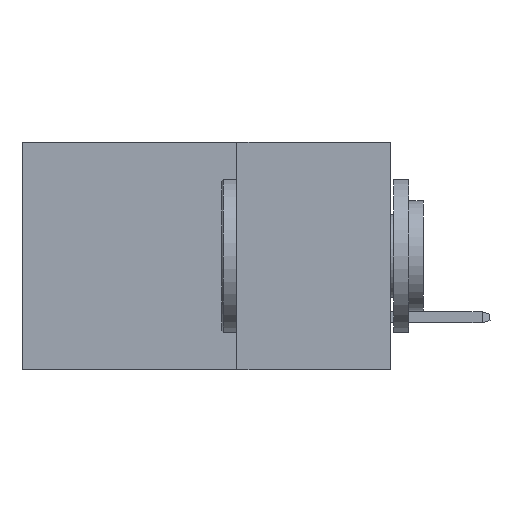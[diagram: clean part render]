
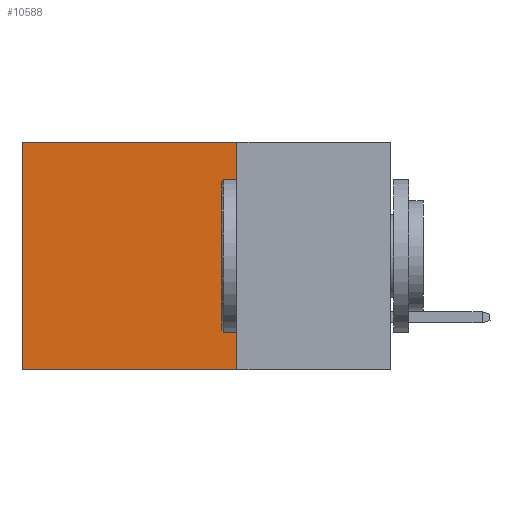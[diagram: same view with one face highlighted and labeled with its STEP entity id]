
A CAD part, left-side view. The second image highlights one B-rep face of the part: STEP entity #10588.
In plain terms, the highlighted planar face has unit normal (-1, 0, 0).
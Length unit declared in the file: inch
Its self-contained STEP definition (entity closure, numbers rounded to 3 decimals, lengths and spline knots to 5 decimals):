
#718 = CARTESIAN_POINT ( 'NONE',  ( 0.2875, 0.6, -0.37 ) ) ;
#888 = VECTOR ( 'NONE', #8191, 39.37008 ) ;
#1905 = VERTEX_POINT ( 'NONE', #718 ) ;
#2585 = DIRECTION ( 'NONE',  ( 0., 0., -1. ) ) ;
#2969 = ORIENTED_EDGE ( 'NONE', *, *, #6044, .F. ) ;
#3338 = VERTEX_POINT ( 'NONE', #7557 ) ;
#3900 = DIRECTION ( 'NONE',  ( 0., 0., -1. ) ) ;
#4353 = LINE ( 'NONE', #6935, #888 ) ;
#5062 = VECTOR ( 'NONE', #14780, 39.37008 ) ;
#5871 = CARTESIAN_POINT ( 'NONE',  ( 0.2875, 0.25, 0. ) ) ;
#6044 = EDGE_CURVE ( 'NONE', #3338, #1905, #4353, .T. ) ;
#6286 = VECTOR ( 'NONE', #3900, 39.37008 ) ;
#6489 = VERTEX_POINT ( 'NONE', #14646 ) ;
#6721 = EDGE_CURVE ( 'NONE', #6489, #3338, #10018, .T. ) ;
#6835 = CARTESIAN_POINT ( 'NONE',  ( 0.2875, 0.6, 0. ) ) ;
#6935 = CARTESIAN_POINT ( 'NONE',  ( 0.2875, 0.25, -0.37 ) ) ;
#7008 = FACE_OUTER_BOUND ( 'NONE', #14664, .T. ) ;
#7557 = CARTESIAN_POINT ( 'NONE',  ( 0.2875, 0.25, -0.37 ) ) ;
#7708 = CARTESIAN_POINT ( 'NONE',  ( 0.2875, 0.6, 0. ) ) ;
#8191 = DIRECTION ( 'NONE',  ( 0., 1., 0. ) ) ;
#8321 = VECTOR ( 'NONE', #10718, 39.37008 ) ;
#9427 = CARTESIAN_POINT ( 'NONE',  ( 0.2875, 0.25, 0. ) ) ;
#10018 = LINE ( 'NONE', #9427, #8321 ) ;
#10390 = LINE ( 'NONE', #7708, #6286 ) ;
#10588 = ADVANCED_FACE ( 'NONE', ( #7008 ), #15439, .F. ) ;
#10629 = LINE ( 'NONE', #5871, #5062 ) ;
#10718 = DIRECTION ( 'NONE',  ( 0., 0., -1. ) ) ;
#11478 = ORIENTED_EDGE ( 'NONE', *, *, #12809, .T. ) ;
#12500 = EDGE_CURVE ( 'NONE', #6489, #14158, #10629, .T. ) ;
#12616 = ORIENTED_EDGE ( 'NONE', *, *, #6721, .F. ) ;
#12809 = EDGE_CURVE ( 'NONE', #14158, #1905, #10390, .T. ) ;
#13103 = DIRECTION ( 'NONE',  ( 1., 0., 0. ) ) ;
#13738 = AXIS2_PLACEMENT_3D ( 'NONE', #14232, #13103, #2585 ) ;
#14158 = VERTEX_POINT ( 'NONE', #6835 ) ;
#14232 = CARTESIAN_POINT ( 'NONE',  ( 0.2875, 0.25, 0. ) ) ;
#14646 = CARTESIAN_POINT ( 'NONE',  ( 0.2875, 0.25, 0. ) ) ;
#14664 = EDGE_LOOP ( 'NONE', ( #11478, #2969, #12616, #16482 ) ) ;
#14780 = DIRECTION ( 'NONE',  ( 0., 1., 0. ) ) ;
#15439 = PLANE ( 'NONE',  #13738 ) ;
#16482 = ORIENTED_EDGE ( 'NONE', *, *, #12500, .T. ) ;
